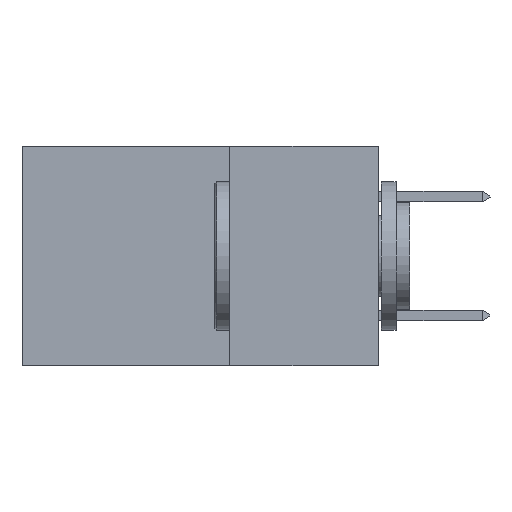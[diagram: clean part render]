
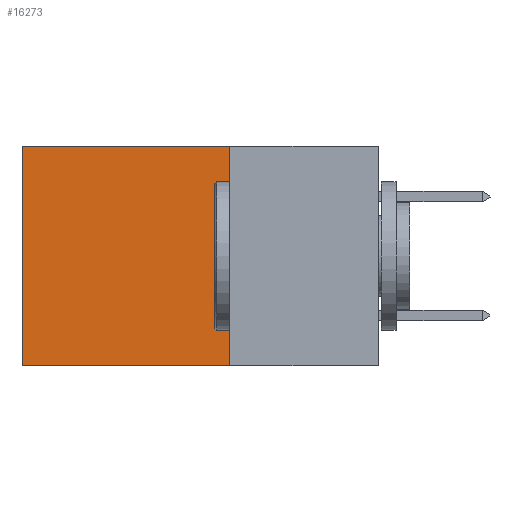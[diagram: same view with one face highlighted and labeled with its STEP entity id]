
A CAD part, left-side view. The second image highlights one B-rep face of the part: STEP entity #16273.
In plain terms, the highlighted planar face has unit normal (-1, 0, 0).
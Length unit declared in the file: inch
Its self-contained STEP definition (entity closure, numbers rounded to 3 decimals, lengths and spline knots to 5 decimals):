
#2 = LINE ( 'NONE', #7348, #8913 ) ;
#289 = VECTOR ( 'NONE', #6322, 39.37008 ) ;
#497 = LINE ( 'NONE', #13404, #1156 ) ;
#790 = VERTEX_POINT ( 'NONE', #3309 ) ;
#1156 = VECTOR ( 'NONE', #14861, 39.37008 ) ;
#1158 = VECTOR ( 'NONE', #12577, 39.37008 ) ;
#2233 = VERTEX_POINT ( 'NONE', #16757 ) ;
#2901 = ORIENTED_EDGE ( 'NONE', *, *, #7112, .F. ) ;
#3300 = EDGE_CURVE ( 'NONE', #2233, #790, #497, .T. ) ;
#3309 = CARTESIAN_POINT ( 'NONE',  ( 0.298, 0.25, -0.37 ) ) ;
#3339 = CARTESIAN_POINT ( 'NONE',  ( 0.298, 0.6, 0. ) ) ;
#3759 = CARTESIAN_POINT ( 'NONE',  ( 0.298, 0.25, 0. ) ) ;
#4060 = LINE ( 'NONE', #3339, #289 ) ;
#5306 = VERTEX_POINT ( 'NONE', #7695 ) ;
#6322 = DIRECTION ( 'NONE',  ( 0., 0., -1. ) ) ;
#6502 = VERTEX_POINT ( 'NONE', #8325 ) ;
#6594 = EDGE_CURVE ( 'NONE', #6502, #5306, #4060, .T. ) ;
#6741 = PLANE ( 'NONE',  #16075 ) ;
#7112 = EDGE_CURVE ( 'NONE', #790, #5306, #11861, .T. ) ;
#7348 = CARTESIAN_POINT ( 'NONE',  ( 0.298, 0.25, 0. ) ) ;
#7695 = CARTESIAN_POINT ( 'NONE',  ( 0.298, 0.6, -0.37 ) ) ;
#7933 = EDGE_CURVE ( 'NONE', #2233, #6502, #2, .T. ) ;
#8311 = CARTESIAN_POINT ( 'NONE',  ( 0.298, 0.25, -0.37 ) ) ;
#8325 = CARTESIAN_POINT ( 'NONE',  ( 0.298, 0.6, 0. ) ) ;
#8913 = VECTOR ( 'NONE', #14484, 39.37008 ) ;
#8937 = ORIENTED_EDGE ( 'NONE', *, *, #7933, .T. ) ;
#9093 = ORIENTED_EDGE ( 'NONE', *, *, #3300, .F. ) ;
#11861 = LINE ( 'NONE', #8311, #1158 ) ;
#12577 = DIRECTION ( 'NONE',  ( 0., 1., 0. ) ) ;
#13404 = CARTESIAN_POINT ( 'NONE',  ( 0.298, 0.25, 0. ) ) ;
#14484 = DIRECTION ( 'NONE',  ( 0., 1., 0. ) ) ;
#14861 = DIRECTION ( 'NONE',  ( 0., 0., -1. ) ) ;
#15834 = ORIENTED_EDGE ( 'NONE', *, *, #6594, .T. ) ;
#16075 = AXIS2_PLACEMENT_3D ( 'NONE', #3759, #17952, #18137 ) ;
#16273 = ADVANCED_FACE ( 'NONE', ( #16802 ), #6741, .F. ) ;
#16757 = CARTESIAN_POINT ( 'NONE',  ( 0.298, 0.25, 0. ) ) ;
#16802 = FACE_OUTER_BOUND ( 'NONE', #17426, .T. ) ;
#17426 = EDGE_LOOP ( 'NONE', ( #15834, #2901, #9093, #8937 ) ) ;
#17952 = DIRECTION ( 'NONE',  ( 1., 0., 0. ) ) ;
#18137 = DIRECTION ( 'NONE',  ( 0., 0., -1. ) ) ;
